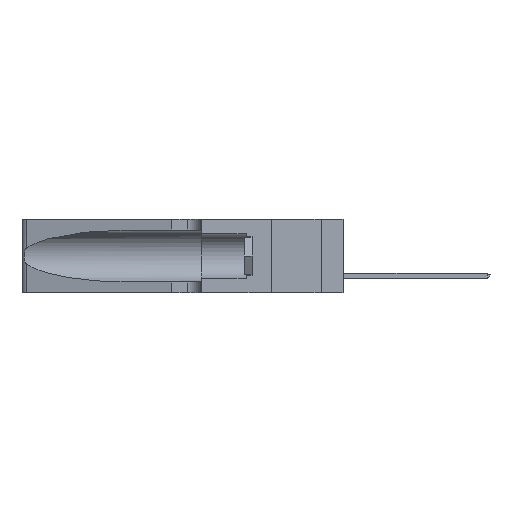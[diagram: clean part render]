
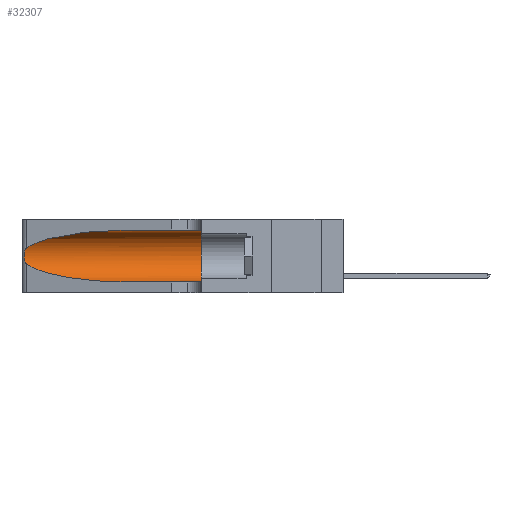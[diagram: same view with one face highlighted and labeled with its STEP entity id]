
A CAD part, left-side view. The second image highlights one B-rep face of the part: STEP entity #32307.
In plain terms, the highlighted cylindrical face has radius 3.308 mm (diameter 6.617 mm), a partial arc.
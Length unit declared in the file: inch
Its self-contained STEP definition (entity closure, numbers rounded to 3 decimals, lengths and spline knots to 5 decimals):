
#59 = VERTEX_POINT ( 'NONE', #19768 ) ;
#667 = ORIENTED_EDGE ( 'NONE', *, *, #19255, .F. ) ;
#710 = DIRECTION ( 'NONE',  ( 0., -1., 0. ) ) ;
#1170 = VERTEX_POINT ( 'NONE', #31741 ) ;
#1190 = CYLINDRICAL_SURFACE ( 'NONE', #26829, 0.13025 ) ;
#1692 =( BOUNDED_CURVE ( )  B_SPLINE_CURVE ( 3, ( #2313, #18850, #27282, #24703 ),
 .UNSPECIFIED., .F., .F. ) 
 B_SPLINE_CURVE_WITH_KNOTS ( ( 4, 4 ),
 ( 1.5708, 2.84003 ),
 .UNSPECIFIED. ) 
 CURVE ( )  GEOMETRIC_REPRESENTATION_ITEM ( )  RATIONAL_B_SPLINE_CURVE ( ( 1., 0.87, 0.87, 1. ) ) 
 REPRESENTATION_ITEM ( '' )  );
#1842 = CARTESIAN_POINT ( 'NONE',  ( 0.25789, 1.23486, 0.15765 ) ) ;
#2313 = CARTESIAN_POINT ( 'NONE',  ( 0.1305, 0.72297, 0.31525 ) ) ;
#3771 = CARTESIAN_POINT ( 'NONE',  ( 0.25555, 1.22994, 0.2215 ) ) ;
#3965 = EDGE_CURVE ( 'NONE', #34712, #1170, #24572, .T. ) ;
#4673 = CARTESIAN_POINT ( 'NONE',  ( 0.25555, 1.22993, 0.14849 ) ) ;
#5406 = CARTESIAN_POINT ( 'NONE',  ( 0.25487, 1.22718, 0.22369 ) ) ;
#5517 = EDGE_CURVE ( 'NONE', #14633, #6427, #1692, .T. ) ;
#5743 = VECTOR ( 'NONE', #10854, 39.37008 ) ;
#6427 = VERTEX_POINT ( 'NONE', #32004 ) ;
#6905 = CARTESIAN_POINT ( 'NONE',  ( 0.25487, 1.22718, 0.14631 ) ) ;
#6961 = CARTESIAN_POINT ( 'NONE',  ( 0.26075, 1.23896, 0.19203 ) ) ;
#7011 = EDGE_LOOP ( 'NONE', ( #28557, #20801, #29769, #26735, #667, #18134 ) ) ;
#7302 = DIRECTION ( 'NONE',  ( 0., -1., 0. ) ) ;
#7838 = FACE_OUTER_BOUND ( 'NONE', #7011, .T. ) ;
#8045 = CARTESIAN_POINT ( 'NONE',  ( 0.25639, 1.23184, 0.21858 ) ) ;
#9186 = CARTESIAN_POINT ( 'NONE',  ( 0.1305, 1.61858, 0.185 ) ) ;
#10170 = CARTESIAN_POINT ( 'NONE',  ( 0.25856, 1.23593, 0.16098 ) ) ;
#10482 = CARTESIAN_POINT ( 'NONE',  ( 0.18966, 0.96281, 0.05475 ) ) ;
#10605 = CARTESIAN_POINT ( 'NONE',  ( 0.1305, 0.72297, 0.05475 ) ) ;
#10854 = DIRECTION ( 'NONE',  ( 0., -1., 0. ) ) ;
#12610 = CARTESIAN_POINT ( 'NONE',  ( 0.26075, 1.23896, 0.178 ) ) ;
#12908 = CARTESIAN_POINT ( 'NONE',  ( 0.1305, 0.72297, 0.31525 ) ) ;
#13131 = VERTEX_POINT ( 'NONE', #6905 ) ;
#13415 = CARTESIAN_POINT ( 'NONE',  ( 0.1305, 1.61858, 0.05475 ) ) ;
#13617 = DIRECTION ( 'NONE',  ( 0., 0., 1. ) ) ;
#13819 = CARTESIAN_POINT ( 'NONE',  ( 0.26018, 1.23835, 0.19895 ) ) ;
#14521 = CARTESIAN_POINT ( 'NONE',  ( 0.1305, 0.72297, 0.05475 ) ) ;
#14540 = CARTESIAN_POINT ( 'NONE',  ( 0.25487, 1.22718, 0.14631 ) ) ;
#14633 = VERTEX_POINT ( 'NONE', #12908 ) ;
#16105 = EDGE_CURVE ( 'NONE', #13131, #34712, #18529, .T. ) ;
#18132 = CARTESIAN_POINT ( 'NONE',  ( 0.25487, 1.22718, 0.14631 ) ) ;
#18134 = ORIENTED_EDGE ( 'NONE', *, *, #28315, .F. ) ;
#18529 =( BOUNDED_CURVE ( )  B_SPLINE_CURVE ( 3, ( #14540, #26040, #10482, #10605 ),
 .UNSPECIFIED., .F., .T. ) 
 B_SPLINE_CURVE_WITH_KNOTS ( ( 4, 4 ),
 ( 3.44316, 4.71239 ),
 .UNSPECIFIED. ) 
 CURVE ( )  GEOMETRIC_REPRESENTATION_ITEM ( )  RATIONAL_B_SPLINE_CURVE ( ( 1., 0.87, 0.87, 1. ) ) 
 REPRESENTATION_ITEM ( '' )  );
#18850 = CARTESIAN_POINT ( 'NONE',  ( 0.18966, 0.96281, 0.31525 ) ) ;
#19255 = EDGE_CURVE ( 'NONE', #59, #1170, #35708, .T. ) ;
#19768 = CARTESIAN_POINT ( 'NONE',  ( 0.1305, 0.35, 0.31525 ) ) ;
#20801 = ORIENTED_EDGE ( 'NONE', *, *, #29478, .T. ) ;
#20817 = LINE ( 'NONE', #35253, #34791 ) ;
#22323 = AXIS2_PLACEMENT_3D ( 'NONE', #26993, #24773, #13617 ) ;
#23130 = DIRECTION ( 'NONE',  ( 0., 0., -1. ) ) ;
#23597 = CARTESIAN_POINT ( 'NONE',  ( 0.25854, 1.2359, 0.20912 ) ) ;
#23816 = CARTESIAN_POINT ( 'NONE',  ( 0.25787, 1.23484, 0.2124 ) ) ;
#24572 = LINE ( 'NONE', #13415, #5743 ) ;
#24703 = CARTESIAN_POINT ( 'NONE',  ( 0.25487, 1.22718, 0.22369 ) ) ;
#24773 = DIRECTION ( 'NONE',  ( 0., 1., 0. ) ) ;
#26040 = CARTESIAN_POINT ( 'NONE',  ( 0.2373, 1.15595, 0.08982 ) ) ;
#26735 = ORIENTED_EDGE ( 'NONE', *, *, #3965, .T. ) ;
#26829 = AXIS2_PLACEMENT_3D ( 'NONE', #9186, #710, #23130 ) ;
#26993 = CARTESIAN_POINT ( 'NONE',  ( 0.1305, 0.35, 0.185 ) ) ;
#27282 = CARTESIAN_POINT ( 'NONE',  ( 0.2373, 1.15595, 0.28018 ) ) ;
#28315 = EDGE_CURVE ( 'NONE', #14633, #59, #20817, .T. ) ;
#28557 = ORIENTED_EDGE ( 'NONE', *, *, #5517, .T. ) ;
#29478 = EDGE_CURVE ( 'NONE', #6427, #13131, #31809, .T. ) ;
#29736 = CARTESIAN_POINT ( 'NONE',  ( 0.26017, 1.23833, 0.17102 ) ) ;
#29769 = ORIENTED_EDGE ( 'NONE', *, *, #16105, .T. ) ;
#31741 = CARTESIAN_POINT ( 'NONE',  ( 0.1305, 0.35, 0.05475 ) ) ;
#31809 = B_SPLINE_CURVE_WITH_KNOTS ( 'NONE', 3,
 ( #5406, #3771, #8045, #23816, #23597, #13819, #6961, #12610, #29736, #10170, #1842, #34828, #4673, #18132 ),
 .UNSPECIFIED., .F., .F.,
 ( 4, 2, 2, 2, 2, 2, 4 ),
 ( 0., 0.00027, 0.00053, 0.00107, 0.0016, 0.00187, 0.00214 ),
 .UNSPECIFIED. ) ;
#32004 = CARTESIAN_POINT ( 'NONE',  ( 0.25487, 1.22718, 0.22369 ) ) ;
#32307 = ADVANCED_FACE ( 'NONE', ( #7838 ), #1190, .F. ) ;
#34712 = VERTEX_POINT ( 'NONE', #14521 ) ;
#34791 = VECTOR ( 'NONE', #7302, 39.37008 ) ;
#34828 = CARTESIAN_POINT ( 'NONE',  ( 0.25639, 1.23186, 0.15144 ) ) ;
#35253 = CARTESIAN_POINT ( 'NONE',  ( 0.1305, 1.61858, 0.31525 ) ) ;
#35708 = CIRCLE ( 'NONE', #22323, 0.13025 ) ;
